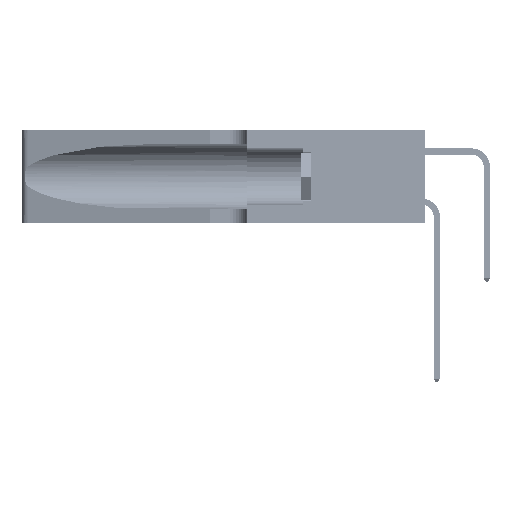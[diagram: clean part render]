
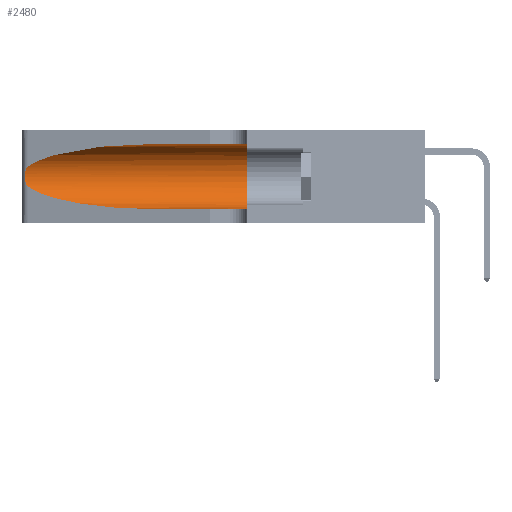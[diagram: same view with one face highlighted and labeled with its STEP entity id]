
A CAD part, left-side view. The second image highlights one B-rep face of the part: STEP entity #2480.
In plain terms, the highlighted cylindrical face has radius 3.308 mm (diameter 6.617 mm), a partial arc.
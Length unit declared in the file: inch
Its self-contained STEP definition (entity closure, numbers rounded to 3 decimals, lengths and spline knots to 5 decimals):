
#1983 = CARTESIAN_POINT ( 'NONE',  ( 0.1305, 1.61858, 0.185 ) ) ;
#2042 = CARTESIAN_POINT ( 'NONE',  ( 0.26017, 1.23833, 0.17102 ) ) ;
#2480 = ADVANCED_FACE ( 'NONE', ( #20086 ), #50247, .F. ) ;
#2929 =( BOUNDED_CURVE ( )  B_SPLINE_CURVE ( 3, ( #50881, #22165, #30505, #5777 ),
 .UNSPECIFIED., .F., .F. ) 
 B_SPLINE_CURVE_WITH_KNOTS ( ( 4, 4 ),
 ( 1.5708, 2.84003 ),
 .UNSPECIFIED. ) 
 CURVE ( )  GEOMETRIC_REPRESENTATION_ITEM ( )  RATIONAL_B_SPLINE_CURVE ( ( 1., 0.87, 0.87, 1. ) ) 
 REPRESENTATION_ITEM ( '' )  );
#3647 = AXIS2_PLACEMENT_3D ( 'NONE', #7965, #36829, #12095 ) ;
#4621 = CARTESIAN_POINT ( 'NONE',  ( 0.1305, 0.35, 0.05475 ) ) ;
#4634 = VERTEX_POINT ( 'NONE', #44273 ) ;
#4918 = VERTEX_POINT ( 'NONE', #45865 ) ;
#5061 = CARTESIAN_POINT ( 'NONE',  ( 0.25487, 1.22718, 0.14631 ) ) ;
#5777 = CARTESIAN_POINT ( 'NONE',  ( 0.25487, 1.22718, 0.22369 ) ) ;
#6147 = CARTESIAN_POINT ( 'NONE',  ( 0.25789, 1.23486, 0.15765 ) ) ;
#6676 = EDGE_LOOP ( 'NONE', ( #47907, #21152, #45630, #33769, #25391, #26907 ) ) ;
#7965 = CARTESIAN_POINT ( 'NONE',  ( 0.1305, 0.35, 0.185 ) ) ;
#10091 = CARTESIAN_POINT ( 'NONE',  ( 0.25487, 1.22718, 0.22369 ) ) ;
#10119 = EDGE_CURVE ( 'NONE', #29467, #33075, #52811, .T. ) ;
#10278 = CARTESIAN_POINT ( 'NONE',  ( 0.25555, 1.22993, 0.14849 ) ) ;
#10824 = CARTESIAN_POINT ( 'NONE',  ( 0.1305, 1.61858, 0.31525 ) ) ;
#10834 = VERTEX_POINT ( 'NONE', #17424 ) ;
#11739 = EDGE_CURVE ( 'NONE', #4918, #4634, #50720, .T. ) ;
#12095 = DIRECTION ( 'NONE',  ( 0., 0., 1. ) ) ;
#12976 = DIRECTION ( 'NONE',  ( 0., -1., 0. ) ) ;
#13110 = EDGE_CURVE ( 'NONE', #4634, #27397, #53141, .T. ) ;
#13431 = EDGE_CURVE ( 'NONE', #4918, #10834, #2929, .T. ) ;
#14396 = DIRECTION ( 'NONE',  ( 0., -1., 0. ) ) ;
#17199 = LINE ( 'NONE', #41771, #26914 ) ;
#17424 = CARTESIAN_POINT ( 'NONE',  ( 0.25487, 1.22718, 0.22369 ) ) ;
#18407 = CARTESIAN_POINT ( 'NONE',  ( 0.25787, 1.23484, 0.2124 ) ) ;
#18522 = DIRECTION ( 'NONE',  ( 0., 0., -1. ) ) ;
#20086 = FACE_OUTER_BOUND ( 'NONE', #6676, .T. ) ;
#21152 = ORIENTED_EDGE ( 'NONE', *, *, #35392, .T. ) ;
#22165 = CARTESIAN_POINT ( 'NONE',  ( 0.18966, 0.96281, 0.31525 ) ) ;
#22542 = CARTESIAN_POINT ( 'NONE',  ( 0.26018, 1.23835, 0.19895 ) ) ;
#25391 = ORIENTED_EDGE ( 'NONE', *, *, #13110, .F. ) ;
#26750 = CARTESIAN_POINT ( 'NONE',  ( 0.26075, 1.23896, 0.178 ) ) ;
#26907 = ORIENTED_EDGE ( 'NONE', *, *, #11739, .F. ) ;
#26914 = VECTOR ( 'NONE', #12976, 39.37008 ) ;
#27397 = VERTEX_POINT ( 'NONE', #4621 ) ;
#29467 = VERTEX_POINT ( 'NONE', #40048 ) ;
#30505 = CARTESIAN_POINT ( 'NONE',  ( 0.2373, 1.15595, 0.28018 ) ) ;
#30885 = CARTESIAN_POINT ( 'NONE',  ( 0.25856, 1.23593, 0.16098 ) ) ;
#33009 = CARTESIAN_POINT ( 'NONE',  ( 0.1305, 0.72297, 0.05475 ) ) ;
#33075 = VERTEX_POINT ( 'NONE', #33009 ) ;
#33710 = B_SPLINE_CURVE_WITH_KNOTS ( 'NONE', 3,
 ( #10091, #34834, #43042, #18407, #47151, #22542, #51262, #26750, #2042, #30885, #6147, #35012, #10278, #39132 ),
 .UNSPECIFIED., .F., .F.,
 ( 4, 2, 2, 2, 2, 2, 4 ),
 ( 0., 0.00027, 0.00053, 0.00107, 0.0016, 0.00187, 0.00214 ),
 .UNSPECIFIED. ) ;
#33769 = ORIENTED_EDGE ( 'NONE', *, *, #51584, .T. ) ;
#33910 = CARTESIAN_POINT ( 'NONE',  ( 0.1305, 0.72297, 0.05475 ) ) ;
#34834 = CARTESIAN_POINT ( 'NONE',  ( 0.25555, 1.22994, 0.2215 ) ) ;
#35012 = CARTESIAN_POINT ( 'NONE',  ( 0.25639, 1.23186, 0.15144 ) ) ;
#35392 = EDGE_CURVE ( 'NONE', #10834, #29467, #33710, .T. ) ;
#36829 = DIRECTION ( 'NONE',  ( 0., 1., 0. ) ) ;
#39132 = CARTESIAN_POINT ( 'NONE',  ( 0.25487, 1.22718, 0.14631 ) ) ;
#39880 = VECTOR ( 'NONE', #43748, 39.37008 ) ;
#40048 = CARTESIAN_POINT ( 'NONE',  ( 0.25487, 1.22718, 0.14631 ) ) ;
#41771 = CARTESIAN_POINT ( 'NONE',  ( 0.1305, 1.61858, 0.05475 ) ) ;
#43042 = CARTESIAN_POINT ( 'NONE',  ( 0.25639, 1.23184, 0.21858 ) ) ;
#43679 = AXIS2_PLACEMENT_3D ( 'NONE', #1983, #14396, #18522 ) ;
#43748 = DIRECTION ( 'NONE',  ( 0., -1., 0. ) ) ;
#44273 = CARTESIAN_POINT ( 'NONE',  ( 0.1305, 0.35, 0.31525 ) ) ;
#45630 = ORIENTED_EDGE ( 'NONE', *, *, #10119, .T. ) ;
#45865 = CARTESIAN_POINT ( 'NONE',  ( 0.1305, 0.72297, 0.31525 ) ) ;
#46053 = CARTESIAN_POINT ( 'NONE',  ( 0.2373, 1.15595, 0.08982 ) ) ;
#47151 = CARTESIAN_POINT ( 'NONE',  ( 0.25854, 1.2359, 0.20912 ) ) ;
#47907 = ORIENTED_EDGE ( 'NONE', *, *, #13431, .T. ) ;
#50151 = CARTESIAN_POINT ( 'NONE',  ( 0.18966, 0.96281, 0.05475 ) ) ;
#50247 = CYLINDRICAL_SURFACE ( 'NONE', #43679, 0.13025 ) ;
#50720 = LINE ( 'NONE', #10824, #39880 ) ;
#50881 = CARTESIAN_POINT ( 'NONE',  ( 0.1305, 0.72297, 0.31525 ) ) ;
#51262 = CARTESIAN_POINT ( 'NONE',  ( 0.26075, 1.23896, 0.19203 ) ) ;
#51584 = EDGE_CURVE ( 'NONE', #33075, #27397, #17199, .T. ) ;
#52811 =( BOUNDED_CURVE ( )  B_SPLINE_CURVE ( 3, ( #5061, #46053, #50151, #33910 ),
 .UNSPECIFIED., .F., .F. ) 
 B_SPLINE_CURVE_WITH_KNOTS ( ( 4, 4 ),
 ( 3.44316, 4.71239 ),
 .UNSPECIFIED. ) 
 CURVE ( )  GEOMETRIC_REPRESENTATION_ITEM ( )  RATIONAL_B_SPLINE_CURVE ( ( 1., 0.87, 0.87, 1. ) ) 
 REPRESENTATION_ITEM ( '' )  );
#53141 = CIRCLE ( 'NONE', #3647, 0.13025 ) ;
